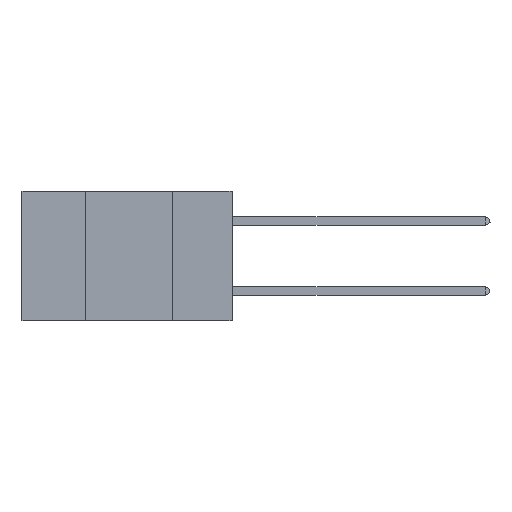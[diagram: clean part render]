
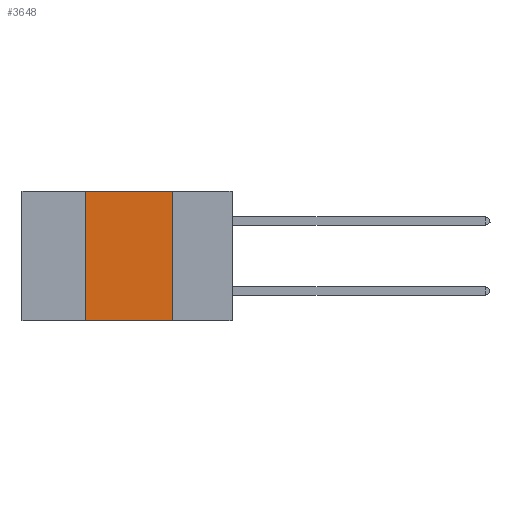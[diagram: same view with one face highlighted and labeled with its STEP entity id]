
A CAD part, left-side view. The second image highlights one B-rep face of the part: STEP entity #3648.
In plain terms, the highlighted planar face has unit normal (-1, 0, 0).
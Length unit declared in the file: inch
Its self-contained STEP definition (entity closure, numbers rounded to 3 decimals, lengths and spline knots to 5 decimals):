
#91 = CARTESIAN_POINT ( 'NONE',  ( 0., 0.6, -0.37 ) ) ;
#709 = EDGE_CURVE ( 'NONE', #1454, #7544, #2741, .T. ) ;
#879 = DIRECTION ( 'NONE',  ( 1., 0., 0. ) ) ;
#911 = LINE ( 'NONE', #4233, #9984 ) ;
#913 = CARTESIAN_POINT ( 'NONE',  ( 0., 0.6, 0. ) ) ;
#1162 = AXIS2_PLACEMENT_3D ( 'NONE', #6616, #879, #7376 ) ;
#1441 = VECTOR ( 'NONE', #6887, 39.37008 ) ;
#1454 = VERTEX_POINT ( 'NONE', #7534 ) ;
#2672 = CARTESIAN_POINT ( 'NONE',  ( 0., 0.17, 0. ) ) ;
#2741 = LINE ( 'NONE', #91, #4431 ) ;
#3408 = DIRECTION ( 'NONE',  ( 0., 0., 1. ) ) ;
#3506 = ORIENTED_EDGE ( 'NONE', *, *, #7294, .F. ) ;
#3648 = ADVANCED_FACE ( 'NONE', ( #7436 ), #4802, .F. ) ;
#4233 = CARTESIAN_POINT ( 'NONE',  ( 0., 0.42, 0. ) ) ;
#4392 = LINE ( 'NONE', #913, #5107 ) ;
#4431 = VECTOR ( 'NONE', #9300, 39.37008 ) ;
#4802 = PLANE ( 'NONE',  #1162 ) ;
#4936 = EDGE_LOOP ( 'NONE', ( #5244, #3506, #8564, #5280 ) ) ;
#5107 = VECTOR ( 'NONE', #7644, 39.37008 ) ;
#5118 = EDGE_CURVE ( 'NONE', #8377, #7544, #7615, .T. ) ;
#5244 = ORIENTED_EDGE ( 'NONE', *, *, #5118, .F. ) ;
#5272 = VERTEX_POINT ( 'NONE', #9488 ) ;
#5280 = ORIENTED_EDGE ( 'NONE', *, *, #709, .T. ) ;
#6119 = EDGE_CURVE ( 'NONE', #1454, #5272, #911, .T. ) ;
#6616 = CARTESIAN_POINT ( 'NONE',  ( 0., 0.6, 0. ) ) ;
#6887 = DIRECTION ( 'NONE',  ( 0., 0., -1. ) ) ;
#7294 = EDGE_CURVE ( 'NONE', #5272, #8377, #4392, .T. ) ;
#7376 = DIRECTION ( 'NONE',  ( 0., 0., -1. ) ) ;
#7436 = FACE_OUTER_BOUND ( 'NONE', #4936, .T. ) ;
#7534 = CARTESIAN_POINT ( 'NONE',  ( 0., 0.42, -0.37 ) ) ;
#7544 = VERTEX_POINT ( 'NONE', #8654 ) ;
#7615 = LINE ( 'NONE', #7708, #1441 ) ;
#7644 = DIRECTION ( 'NONE',  ( 0., -1., 0. ) ) ;
#7708 = CARTESIAN_POINT ( 'NONE',  ( 0., 0.17, 0. ) ) ;
#8377 = VERTEX_POINT ( 'NONE', #2672 ) ;
#8564 = ORIENTED_EDGE ( 'NONE', *, *, #6119, .F. ) ;
#8654 = CARTESIAN_POINT ( 'NONE',  ( 0., 0.17, -0.37 ) ) ;
#9300 = DIRECTION ( 'NONE',  ( 0., -1., 0. ) ) ;
#9488 = CARTESIAN_POINT ( 'NONE',  ( 0., 0.42, 0. ) ) ;
#9984 = VECTOR ( 'NONE', #3408, 39.37008 ) ;
